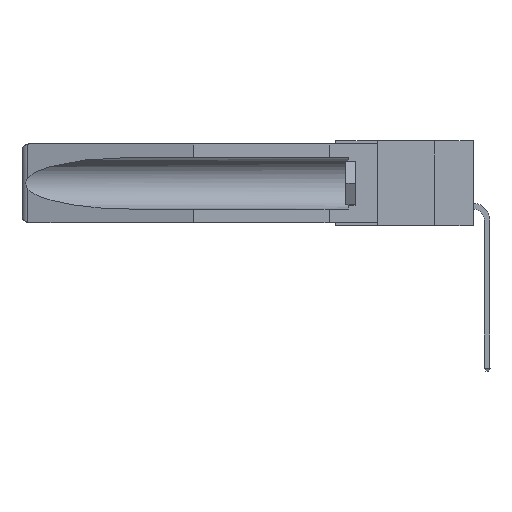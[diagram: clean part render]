
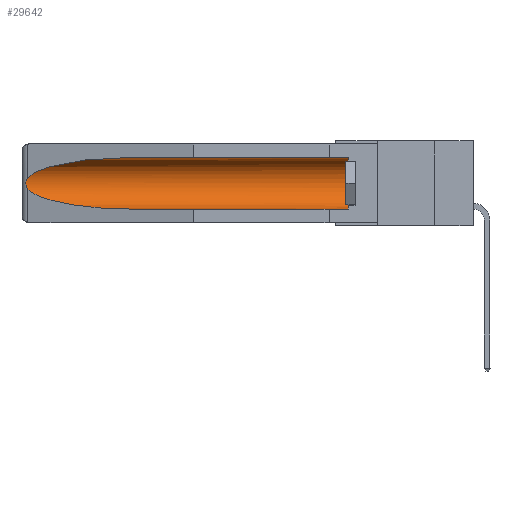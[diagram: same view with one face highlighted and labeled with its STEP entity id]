
A CAD part, left-side view. The second image highlights one B-rep face of the part: STEP entity #29642.
In plain terms, the highlighted cylindrical face has radius 2.857 mm (diameter 5.715 mm), a partial arc.
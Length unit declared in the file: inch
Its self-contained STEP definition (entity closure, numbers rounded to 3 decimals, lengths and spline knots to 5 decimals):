
#80 = CARTESIAN_POINT ( 'NONE',  ( 0.155, 0.126, -0.284 ) ) ;
#2220 =( BOUNDED_CURVE ( )  B_SPLINE_CURVE ( 3, ( #25105, #17967, #12758, #30083 ),
 .UNSPECIFIED., .F., .F. ) 
 B_SPLINE_CURVE_WITH_KNOTS ( ( 4, 4 ),
 ( 4.71239, 6.08839 ),
 .UNSPECIFIED. ) 
 CURVE ( )  GEOMETRIC_REPRESENTATION_ITEM ( )  RATIONAL_B_SPLINE_CURVE ( ( 1., 0.848, 0.848, 1. ) ) 
 REPRESENTATION_ITEM ( '' )  );
#2430 = ORIENTED_EDGE ( 'NONE', *, *, #8330, .T. ) ;
#2495 = CARTESIAN_POINT ( 'NONE',  ( 0.155, 1.07973, -0.284 ) ) ;
#2515 = DIRECTION ( 'NONE',  ( 0., 1., 0. ) ) ;
#3167 = CARTESIAN_POINT ( 'NONE',  ( 0.2675, 1.53308, -0.17534 ) ) ;
#3915 = EDGE_CURVE ( 'NONE', #9814, #9632, #19365, .T. ) ;
#3919 = AXIS2_PLACEMENT_3D ( 'NONE', #24735, #2515, #27408 ) ;
#3998 =( BOUNDED_CURVE ( )  B_SPLINE_CURVE ( 3, ( #19736, #9660, #14871, #2495 ),
 .UNSPECIFIED., .F., .F. ) 
 B_SPLINE_CURVE_WITH_KNOTS ( ( 4, 4 ),
 ( 0.1948, 1.5708 ),
 .UNSPECIFIED. ) 
 CURVE ( )  GEOMETRIC_REPRESENTATION_ITEM ( )  RATIONAL_B_SPLINE_CURVE ( ( 1., 0.848, 0.848, 1. ) ) 
 REPRESENTATION_ITEM ( '' )  );
#4034 = ORIENTED_EDGE ( 'NONE', *, *, #3915, .T. ) ;
#4523 = CARTESIAN_POINT ( 'NONE',  ( 0.155, 1.07973, -0.284 ) ) ;
#4987 = CARTESIAN_POINT ( 'NONE',  ( 0.155, 1.07973, -0.059 ) ) ;
#7239 = ORIENTED_EDGE ( 'NONE', *, *, #28624, .T. ) ;
#7448 = CIRCLE ( 'NONE', #13733, 0.1125 ) ;
#7466 = CARTESIAN_POINT ( 'NONE',  ( 0.26537, 1.52718, -0.19328 ) ) ;
#7599 = ORIENTED_EDGE ( 'NONE', *, *, #22125, .T. ) ;
#8042 = CARTESIAN_POINT ( 'NONE',  ( 0.26537, 1.52718, -0.14972 ) ) ;
#8330 = EDGE_CURVE ( 'NONE', #28991, #9814, #7448, .T. ) ;
#8721 = VECTOR ( 'NONE', #15992, 39.37008 ) ;
#9632 = VERTEX_POINT ( 'NONE', #4987 ) ;
#9660 = CARTESIAN_POINT ( 'NONE',  ( 0.25451, 1.48313, -0.24835 ) ) ;
#9814 = VERTEX_POINT ( 'NONE', #21196 ) ;
#10653 = CARTESIAN_POINT ( 'NONE',  ( 0.26537, 1.52718, -0.19328 ) ) ;
#12334 = CYLINDRICAL_SURFACE ( 'NONE', #3919, 0.1125 ) ;
#12758 = CARTESIAN_POINT ( 'NONE',  ( 0.25451, 1.48313, -0.09465 ) ) ;
#12925 = CARTESIAN_POINT ( 'NONE',  ( 0.26597, 1.52961, -0.15275 ) ) ;
#13088 = DIRECTION ( 'NONE',  ( 0., 1., 0. ) ) ;
#13733 = AXIS2_PLACEMENT_3D ( 'NONE', #19776, #29737, #15018 ) ;
#14871 = CARTESIAN_POINT ( 'NONE',  ( 0.21114, 1.30732, -0.284 ) ) ;
#15018 = DIRECTION ( 'NONE',  ( 0., 0., 1. ) ) ;
#15379 = CARTESIAN_POINT ( 'NONE',  ( 0.155, -0.30754, -0.059 ) ) ;
#15461 = VERTEX_POINT ( 'NONE', #20881 ) ;
#15992 = DIRECTION ( 'NONE',  ( 0., 1., 0. ) ) ;
#16534 = B_SPLINE_CURVE_WITH_KNOTS ( 'NONE', 3,
 ( #8042, #12925, #22784, #22986, #27948, #3167, #20512, #28058, #25688, #10653 ),
 .UNSPECIFIED., .F., .F.,
 ( 4, 2, 2, 2, 4 ),
 ( 0., 0.00029, 0.00058, 0.00087, 0.00117 ),
 .UNSPECIFIED. ) ;
#17967 = CARTESIAN_POINT ( 'NONE',  ( 0.21114, 1.30732, -0.059 ) ) ;
#19365 = LINE ( 'NONE', #15379, #29422 ) ;
#19736 = CARTESIAN_POINT ( 'NONE',  ( 0.26537, 1.52718, -0.19328 ) ) ;
#19776 = CARTESIAN_POINT ( 'NONE',  ( 0.155, 0.126, -0.1715 ) ) ;
#20512 = CARTESIAN_POINT ( 'NONE',  ( 0.2673, 1.53269, -0.17917 ) ) ;
#20881 = CARTESIAN_POINT ( 'NONE',  ( 0.26537, 1.52718, -0.14972 ) ) ;
#21196 = CARTESIAN_POINT ( 'NONE',  ( 0.155, 0.126, -0.059 ) ) ;
#22125 = EDGE_CURVE ( 'NONE', #15461, #24411, #16534, .T. ) ;
#22543 = EDGE_CURVE ( 'NONE', #24411, #26993, #3998, .T. ) ;
#22784 = CARTESIAN_POINT ( 'NONE',  ( 0.26654, 1.53092, -0.15636 ) ) ;
#22986 = CARTESIAN_POINT ( 'NONE',  ( 0.2673, 1.5327, -0.16383 ) ) ;
#23684 = CARTESIAN_POINT ( 'NONE',  ( 0.155, -0.30754, -0.284 ) ) ;
#23759 = ORIENTED_EDGE ( 'NONE', *, *, #22543, .T. ) ;
#24411 = VERTEX_POINT ( 'NONE', #7466 ) ;
#24735 = CARTESIAN_POINT ( 'NONE',  ( 0.155, -0.30754, -0.1715 ) ) ;
#25105 = CARTESIAN_POINT ( 'NONE',  ( 0.155, 1.07973, -0.059 ) ) ;
#25688 = CARTESIAN_POINT ( 'NONE',  ( 0.26597, 1.5296, -0.19026 ) ) ;
#26290 = FACE_OUTER_BOUND ( 'NONE', #29070, .T. ) ;
#26555 = LINE ( 'NONE', #23684, #8721 ) ;
#26674 = ORIENTED_EDGE ( 'NONE', *, *, #32034, .F. ) ;
#26993 = VERTEX_POINT ( 'NONE', #4523 ) ;
#27408 = DIRECTION ( 'NONE',  ( 0., 0., 1. ) ) ;
#27948 = CARTESIAN_POINT ( 'NONE',  ( 0.2675, 1.53308, -0.16763 ) ) ;
#28058 = CARTESIAN_POINT ( 'NONE',  ( 0.26655, 1.53094, -0.18657 ) ) ;
#28624 = EDGE_CURVE ( 'NONE', #9632, #15461, #2220, .T. ) ;
#28991 = VERTEX_POINT ( 'NONE', #80 ) ;
#29070 = EDGE_LOOP ( 'NONE', ( #7239, #7599, #23759, #26674, #2430, #4034 ) ) ;
#29422 = VECTOR ( 'NONE', #13088, 39.37008 ) ;
#29642 = ADVANCED_FACE ( 'NONE', ( #26290 ), #12334, .F. ) ;
#29737 = DIRECTION ( 'NONE',  ( 0., -1., 0. ) ) ;
#30083 = CARTESIAN_POINT ( 'NONE',  ( 0.26537, 1.52718, -0.14972 ) ) ;
#32034 = EDGE_CURVE ( 'NONE', #28991, #26993, #26555, .T. ) ;
